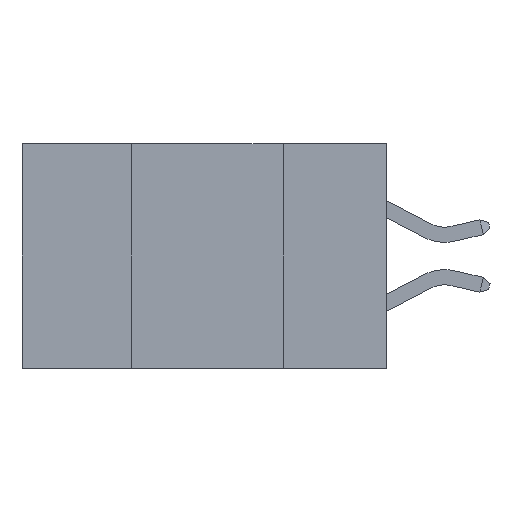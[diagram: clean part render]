
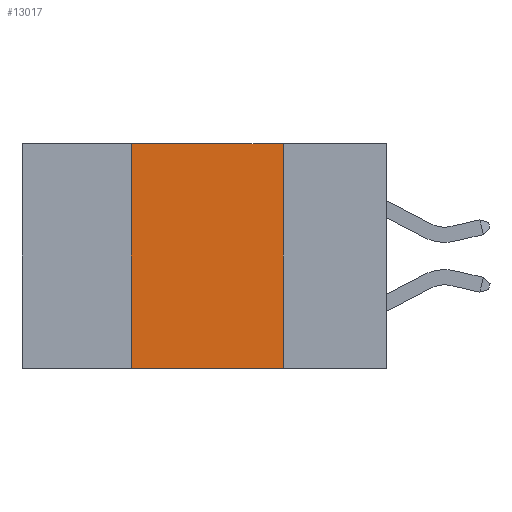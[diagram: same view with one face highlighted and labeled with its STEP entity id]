
A CAD part, left-side view. The second image highlights one B-rep face of the part: STEP entity #13017.
In plain terms, the highlighted planar face has unit normal (-1, 0, 0).
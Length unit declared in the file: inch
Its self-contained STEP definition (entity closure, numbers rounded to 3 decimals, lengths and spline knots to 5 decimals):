
#840 = VECTOR ( 'NONE', #8284, 39.37008 ) ;
#1635 = VECTOR ( 'NONE', #18722, 39.37008 ) ;
#1907 = CARTESIAN_POINT ( 'NONE',  ( 0., 0.42, 0. ) ) ;
#2577 = ORIENTED_EDGE ( 'NONE', *, *, #8493, .F. ) ;
#3842 = VERTEX_POINT ( 'NONE', #23125 ) ;
#4549 = DIRECTION ( 'NONE',  ( 0., -1., 0. ) ) ;
#5833 = CARTESIAN_POINT ( 'NONE',  ( 0., 0.6, 0. ) ) ;
#6801 = CARTESIAN_POINT ( 'NONE',  ( 0., 0.6, 0. ) ) ;
#7705 = ORIENTED_EDGE ( 'NONE', *, *, #17968, .F. ) ;
#8284 = DIRECTION ( 'NONE',  ( 0., -1., 0. ) ) ;
#8493 = EDGE_CURVE ( 'NONE', #3842, #19542, #22466, .T. ) ;
#8698 = EDGE_CURVE ( 'NONE', #11712, #3842, #24368, .T. ) ;
#9164 = CARTESIAN_POINT ( 'NONE',  ( 0., 0.17, 0. ) ) ;
#9602 = DIRECTION ( 'NONE',  ( 1., 0., 0. ) ) ;
#11712 = VERTEX_POINT ( 'NONE', #26285 ) ;
#11838 = PLANE ( 'NONE',  #24160 ) ;
#13017 = ADVANCED_FACE ( 'NONE', ( #17728 ), #11838, .F. ) ;
#13113 = LINE ( 'NONE', #9164, #1635 ) ;
#13524 = VECTOR ( 'NONE', #4549, 39.37008 ) ;
#13811 = CARTESIAN_POINT ( 'NONE',  ( 0., 0.17, 0. ) ) ;
#14441 = EDGE_CURVE ( 'NONE', #11712, #20657, #20297, .T. ) ;
#17494 = ORIENTED_EDGE ( 'NONE', *, *, #14441, .T. ) ;
#17728 = FACE_OUTER_BOUND ( 'NONE', #19145, .T. ) ;
#17968 = EDGE_CURVE ( 'NONE', #19542, #20657, #13113, .T. ) ;
#18259 = CARTESIAN_POINT ( 'NONE',  ( 0., 0.17, -0.37 ) ) ;
#18722 = DIRECTION ( 'NONE',  ( 0., 0., -1. ) ) ;
#19145 = EDGE_LOOP ( 'NONE', ( #7705, #2577, #24342, #17494 ) ) ;
#19542 = VERTEX_POINT ( 'NONE', #13811 ) ;
#20297 = LINE ( 'NONE', #22311, #840 ) ;
#20657 = VERTEX_POINT ( 'NONE', #18259 ) ;
#22117 = DIRECTION ( 'NONE',  ( 0., 0., -1. ) ) ;
#22311 = CARTESIAN_POINT ( 'NONE',  ( 0., 0.6, -0.37 ) ) ;
#22466 = LINE ( 'NONE', #6801, #13524 ) ;
#23125 = CARTESIAN_POINT ( 'NONE',  ( 0., 0.42, 0. ) ) ;
#24158 = DIRECTION ( 'NONE',  ( 0., 0., 1. ) ) ;
#24160 = AXIS2_PLACEMENT_3D ( 'NONE', #5833, #9602, #22117 ) ;
#24342 = ORIENTED_EDGE ( 'NONE', *, *, #8698, .F. ) ;
#24368 = LINE ( 'NONE', #1907, #25673 ) ;
#25673 = VECTOR ( 'NONE', #24158, 39.37008 ) ;
#26285 = CARTESIAN_POINT ( 'NONE',  ( 0., 0.42, -0.37 ) ) ;
